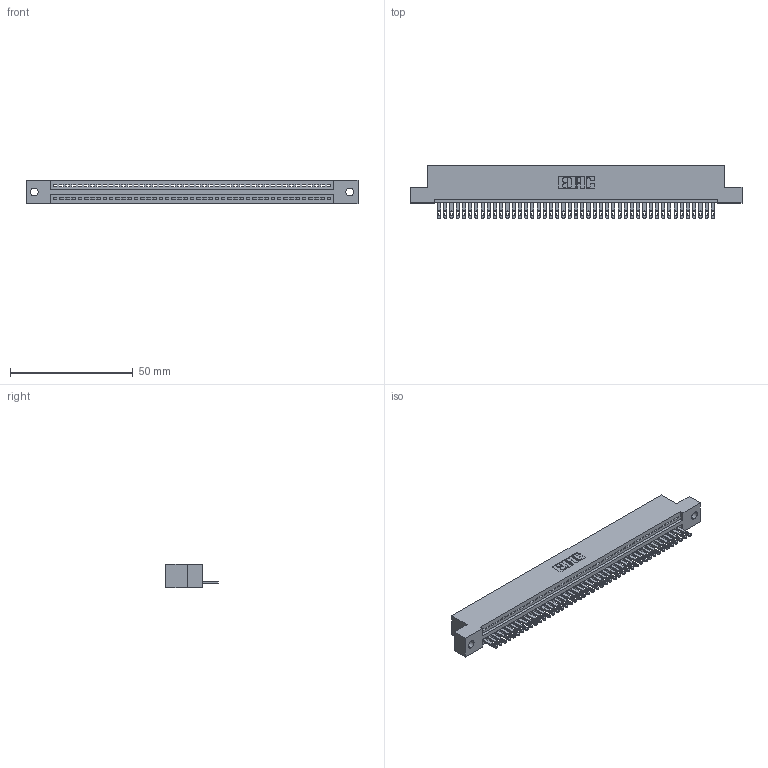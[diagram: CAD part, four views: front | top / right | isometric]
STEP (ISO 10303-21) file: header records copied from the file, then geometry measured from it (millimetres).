
FILE_DESCRIPTION (( 'STEP AP203' ), '1' );
FILE_NAME ('895-045-500-102.STEP', '2020-09-27T03:53:11', ( '' ), ( '' ), 'SwSTEP 2.0', 'SolidWorks 2020', '' );
FILE_SCHEMA (( 'CONFIG_CONTROL_DESIGN' ));
Length unit declared in the file: inch
Products named in the file (3): 845 Part_Flush Mounting Lugs - 0.128 Dia; 345-292-001_345-293-100; 895-045-500-102
Assembly tree (46 placements, depth 2):
  895-045-500-102
    845 Part_Flush Mounting Lugs - 0.128 Dia
    345-292-001_345-293-100  x45
Bounding box: 135.51 x 21.51 x 9.4 mm (x, y, z)
Volume: 12886.5 mm3; surface area: 16995.4 mm2
Topology: 46 solids, 46 shells, 2556 faces, 7901 edges, 5266 vertices
Faces by surface type: plane 1610, cylinder 946
Entity records: 33397 total; most frequent: CARTESIAN_POINT 5791, ORIENTED_EDGE 5770, DIRECTION 5055, EDGE_CURVE 2885, LINE 2569, VECTOR 2569, VERTEX_POINT 1922, AXIS2_PLACEMENT_3D 1243
